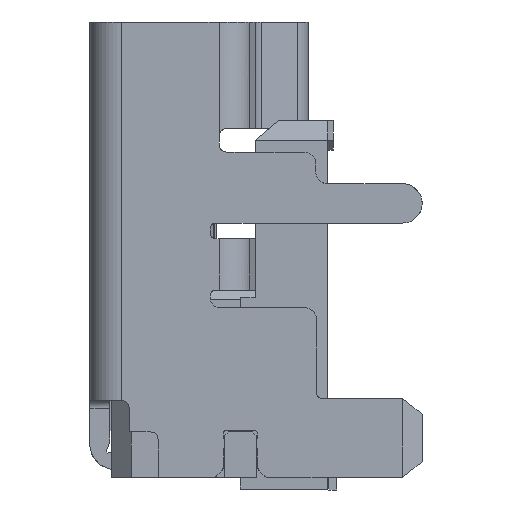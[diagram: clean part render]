
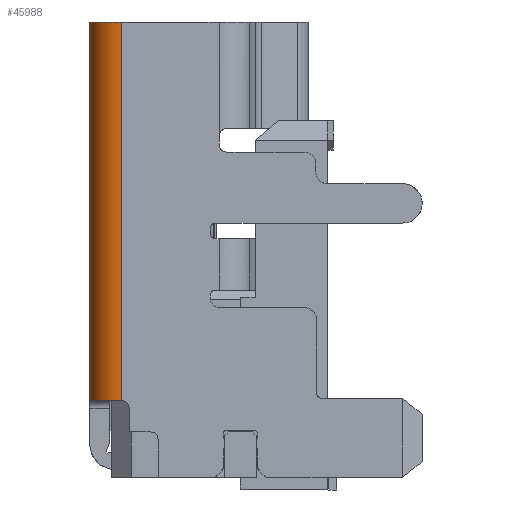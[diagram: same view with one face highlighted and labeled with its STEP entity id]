
A CAD part, left-side view. The second image highlights one B-rep face of the part: STEP entity #45988.
In plain terms, the highlighted cylindrical face has radius 0.8 mm (diameter 1.6 mm), a partial arc.
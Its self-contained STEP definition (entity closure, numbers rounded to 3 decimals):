
#1036 = ORIENTED_EDGE ( 'NONE', *, *, #11747, .T. ) ;
#1310 = CARTESIAN_POINT ( 'NONE',  ( -6.7, 0.525, -7.1 ) ) ;
#1792 = VERTEX_POINT ( 'NONE', #27888 ) ;
#2049 = CARTESIAN_POINT ( 'NONE',  ( -7.5, -0.066, 2.5 ) ) ;
#3211 = CYLINDRICAL_SURFACE ( 'NONE', #27781, 0.8 ) ;
#4283 = EDGE_CURVE ( 'NONE', #51152, #1792, #4946, .T. ) ;
#4946 = B_SPLINE_CURVE_WITH_KNOTS ( 'NONE', 3,
 ( #57480, #52141, #28788, #53070, #38238, #24032 ),
 .UNSPECIFIED., .F., .F.,
 ( 4, 2, 4 ),
 ( 0., 0.5, 1. ),
 .UNSPECIFIED. ) ;
#8427 = VECTOR ( 'NONE', #45313, 1000. ) ;
#11747 = EDGE_CURVE ( 'NONE', #52669, #51152, #54798, .T. ) ;
#15946 = LINE ( 'NONE', #49055, #16601 ) ;
#16601 = VECTOR ( 'NONE', #25074, 1000. ) ;
#16752 = ORIENTED_EDGE ( 'NONE', *, *, #4283, .T. ) ;
#20312 = CARTESIAN_POINT ( 'NONE',  ( -6.7, 0.525, 2.5 ) ) ;
#20603 = EDGE_LOOP ( 'NONE', ( #1036, #16752, #30714, #20836 ) ) ;
#20836 = ORIENTED_EDGE ( 'NONE', *, *, #29426, .T. ) ;
#24032 = CARTESIAN_POINT ( 'NONE',  ( -7.5, -0.275, -7.1 ) ) ;
#25074 = DIRECTION ( 'NONE',  ( 0., 0., -1. ) ) ;
#27228 = CARTESIAN_POINT ( 'NONE',  ( -7.5, -0.275, 2.5 ) ) ;
#27781 = AXIS2_PLACEMENT_3D ( 'NONE', #61875, #31624, #32552 ) ;
#27888 = CARTESIAN_POINT ( 'NONE',  ( -7.5, -0.275, -7.1 ) ) ;
#28788 = CARTESIAN_POINT ( 'NONE',  ( -7.118, 0.439, -7.1 ) ) ;
#29426 = EDGE_CURVE ( 'NONE', #44923, #52669, #62058, .T. ) ;
#30714 = ORIENTED_EDGE ( 'NONE', *, *, #37244, .F. ) ;
#31624 = DIRECTION ( 'NONE',  ( 0., 0., -1. ) ) ;
#31945 = FACE_OUTER_BOUND ( 'NONE', #20603, .T. ) ;
#32552 = DIRECTION ( 'NONE',  ( 0., 1., 0. ) ) ;
#35505 = CARTESIAN_POINT ( 'NONE',  ( -7.118, 0.439, 2.5 ) ) ;
#36137 = CARTESIAN_POINT ( 'NONE',  ( -7.5, -0.275, 2.5 ) ) ;
#37244 = EDGE_CURVE ( 'NONE', #44923, #1792, #15946, .T. ) ;
#38238 = CARTESIAN_POINT ( 'NONE',  ( -7.5, -0.066, -7.1 ) ) ;
#40227 = CARTESIAN_POINT ( 'NONE',  ( -7.414, 0.143, 2.5 ) ) ;
#40907 = CARTESIAN_POINT ( 'NONE',  ( -6.7, 0.525, -2.3 ) ) ;
#42478 = CARTESIAN_POINT ( 'NONE',  ( -6.7, 0.525, 2.5 ) ) ;
#44923 = VERTEX_POINT ( 'NONE', #27228 ) ;
#45251 = CARTESIAN_POINT ( 'NONE',  ( -6.909, 0.525, 2.5 ) ) ;
#45313 = DIRECTION ( 'NONE',  ( 0., 0., -1. ) ) ;
#45988 = ADVANCED_FACE ( 'NONE', ( #31945 ), #3211, .T. ) ;
#49055 = CARTESIAN_POINT ( 'NONE',  ( -7.5, -0.275, -3.275 ) ) ;
#51152 = VERTEX_POINT ( 'NONE', #1310 ) ;
#52141 = CARTESIAN_POINT ( 'NONE',  ( -6.909, 0.525, -7.1 ) ) ;
#52669 = VERTEX_POINT ( 'NONE', #42478 ) ;
#53070 = CARTESIAN_POINT ( 'NONE',  ( -7.414, 0.143, -7.1 ) ) ;
#54798 = LINE ( 'NONE', #40907, #8427 ) ;
#57480 = CARTESIAN_POINT ( 'NONE',  ( -6.7, 0.525, -7.1 ) ) ;
#61875 = CARTESIAN_POINT ( 'NONE',  ( -6.7, -0.275, 3.46 ) ) ;
#62058 = B_SPLINE_CURVE_WITH_KNOTS ( 'NONE', 3,
 ( #36137, #2049, #40227, #35505, #45251, #20312 ),
 .UNSPECIFIED., .F., .F.,
 ( 4, 2, 4 ),
 ( 0., 0.5, 1. ),
 .UNSPECIFIED. ) ;
